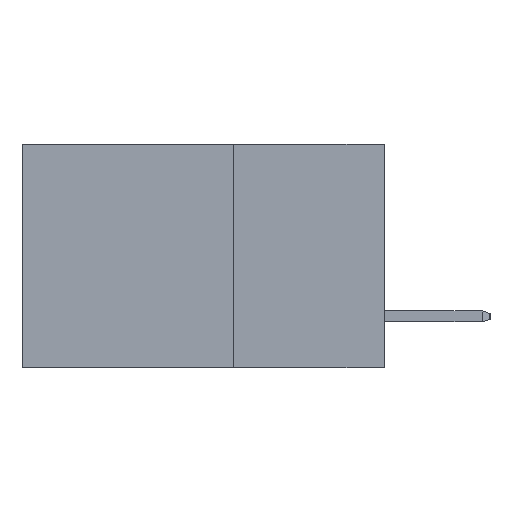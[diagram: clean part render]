
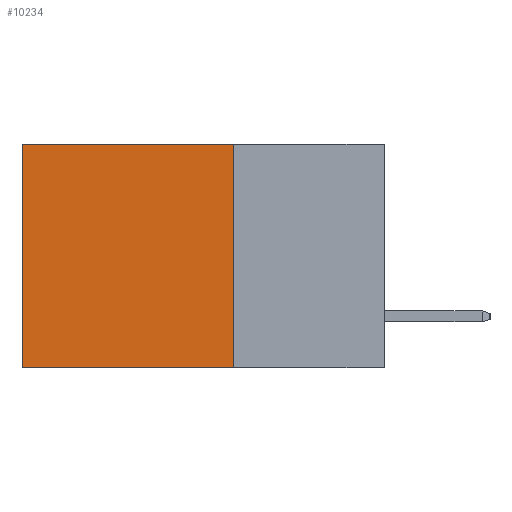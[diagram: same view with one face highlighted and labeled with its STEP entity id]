
A CAD part, left-side view. The second image highlights one B-rep face of the part: STEP entity #10234.
In plain terms, the highlighted planar face has unit normal (-1, 0, 0).
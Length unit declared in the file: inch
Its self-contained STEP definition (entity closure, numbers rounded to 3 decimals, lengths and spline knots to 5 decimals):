
#28 = DIRECTION ( 'NONE',  ( 0., 0., -1. ) ) ;
#556 = LINE ( 'NONE', #4849, #12118 ) ;
#695 = EDGE_CURVE ( 'NONE', #13923, #1572, #13438, .T. ) ;
#1376 = VERTEX_POINT ( 'NONE', #3131 ) ;
#1572 = VERTEX_POINT ( 'NONE', #11538 ) ;
#1897 = AXIS2_PLACEMENT_3D ( 'NONE', #3465, #4633, #11831 ) ;
#2002 = ORIENTED_EDGE ( 'NONE', *, *, #4927, .T. ) ;
#3131 = CARTESIAN_POINT ( 'NONE',  ( 0.2615, 0.6, -0.37 ) ) ;
#3465 = CARTESIAN_POINT ( 'NONE',  ( 0.2615, 0.25, -0.37 ) ) ;
#4168 = LINE ( 'NONE', #12021, #9768 ) ;
#4215 = EDGE_CURVE ( 'NONE', #1572, #1376, #556, .T. ) ;
#4591 = DIRECTION ( 'NONE',  ( 0., 1., 0. ) ) ;
#4633 = DIRECTION ( 'NONE',  ( 1., 0., 0. ) ) ;
#4849 = CARTESIAN_POINT ( 'NONE',  ( 0.2615, 0.25, -0.37 ) ) ;
#4927 = EDGE_CURVE ( 'NONE', #6583, #1376, #4168, .T. ) ;
#5134 = VECTOR ( 'NONE', #4591, 39.37008 ) ;
#5245 = EDGE_LOOP ( 'NONE', ( #2002, #12628, #10434, #13597 ) ) ;
#5278 = VECTOR ( 'NONE', #6221, 39.37008 ) ;
#5476 = FACE_OUTER_BOUND ( 'NONE', #5245, .T. ) ;
#5574 = CARTESIAN_POINT ( 'NONE',  ( 0.2615, 0.25, -0.37 ) ) ;
#6221 = DIRECTION ( 'NONE',  ( 0., 0., -1. ) ) ;
#6331 = CARTESIAN_POINT ( 'NONE',  ( 0.2615, 0.25, 0. ) ) ;
#6583 = VERTEX_POINT ( 'NONE', #8057 ) ;
#8057 = CARTESIAN_POINT ( 'NONE',  ( 0.2615, 0.6, 0. ) ) ;
#8082 = DIRECTION ( 'NONE',  ( 0., 1., 0. ) ) ;
#9768 = VECTOR ( 'NONE', #28, 39.37008 ) ;
#9801 = CARTESIAN_POINT ( 'NONE',  ( 0.2615, 0.25, 0. ) ) ;
#9851 = PLANE ( 'NONE',  #1897 ) ;
#10203 = EDGE_CURVE ( 'NONE', #13923, #6583, #13892, .T. ) ;
#10234 = ADVANCED_FACE ( 'NONE', ( #5476 ), #9851, .F. ) ;
#10434 = ORIENTED_EDGE ( 'NONE', *, *, #695, .F. ) ;
#11538 = CARTESIAN_POINT ( 'NONE',  ( 0.2615, 0.25, -0.37 ) ) ;
#11831 = DIRECTION ( 'NONE',  ( 0., 0., -1. ) ) ;
#12021 = CARTESIAN_POINT ( 'NONE',  ( 0.2615, 0.6, -0.37 ) ) ;
#12118 = VECTOR ( 'NONE', #8082, 39.37008 ) ;
#12628 = ORIENTED_EDGE ( 'NONE', *, *, #4215, .F. ) ;
#13438 = LINE ( 'NONE', #5574, #5278 ) ;
#13597 = ORIENTED_EDGE ( 'NONE', *, *, #10203, .T. ) ;
#13892 = LINE ( 'NONE', #9801, #5134 ) ;
#13923 = VERTEX_POINT ( 'NONE', #6331 ) ;
